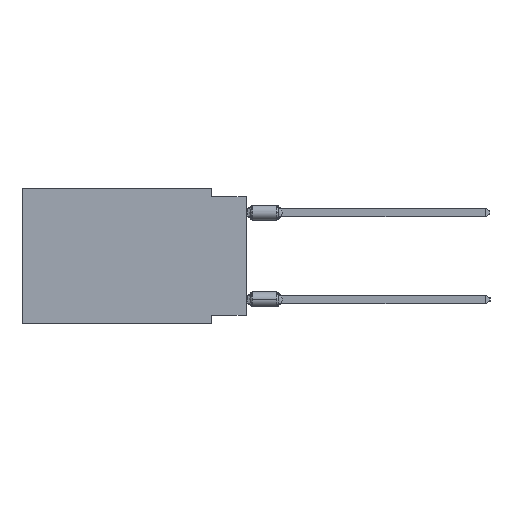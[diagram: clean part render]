
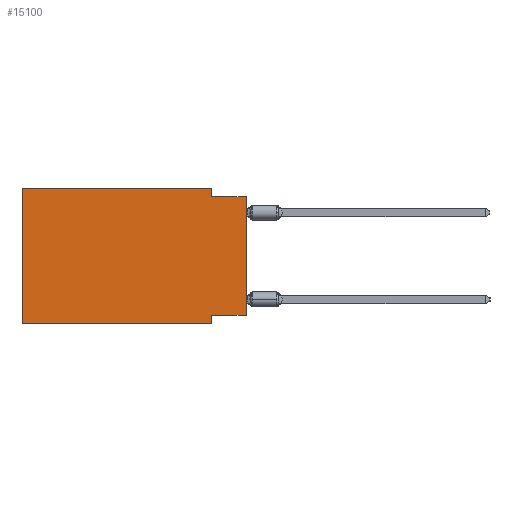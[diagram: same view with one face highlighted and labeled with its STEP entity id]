
A CAD part, left-side view. The second image highlights one B-rep face of the part: STEP entity #15100.
In plain terms, the highlighted planar face has unit normal (-1, 0, 0).
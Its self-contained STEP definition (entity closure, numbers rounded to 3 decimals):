
#609 = LINE ( 'NONE', #11092, #6126 ) ;
#637 = LINE ( 'NONE', #15640, #22141 ) ;
#1046 = VERTEX_POINT ( 'NONE', #30726 ) ;
#1309 = DIRECTION ( 'NONE',  ( 0., 0., 1. ) ) ;
#1723 = LINE ( 'NONE', #22529, #19626 ) ;
#3547 = VERTEX_POINT ( 'NONE', #27599 ) ;
#3715 = EDGE_CURVE ( 'NONE', #22138, #19962, #637, .T. ) ;
#4465 = DIRECTION ( 'NONE',  ( 0., -1., 0. ) ) ;
#4510 = VECTOR ( 'NONE', #1309, 1000. ) ;
#5975 = ORIENTED_EDGE ( 'NONE', *, *, #26621, .F. ) ;
#6126 = VECTOR ( 'NONE', #20151, 1000. ) ;
#6165 = DIRECTION ( 'NONE',  ( 0., 1., 0. ) ) ;
#6294 = EDGE_CURVE ( 'NONE', #22138, #8453, #24699, .T. ) ;
#7339 = ORIENTED_EDGE ( 'NONE', *, *, #3715, .T. ) ;
#7971 = EDGE_CURVE ( 'NONE', #3547, #11430, #24316, .T. ) ;
#8399 = LINE ( 'NONE', #32108, #19657 ) ;
#8453 = VERTEX_POINT ( 'NONE', #26685 ) ;
#9452 = ORIENTED_EDGE ( 'NONE', *, *, #14003, .F. ) ;
#10922 = ORIENTED_EDGE ( 'NONE', *, *, #25157, .F. ) ;
#11092 = CARTESIAN_POINT ( 'NONE',  ( 0., 0., 0. ) ) ;
#11134 = CARTESIAN_POINT ( 'NONE',  ( 0., 16.383, 0. ) ) ;
#11430 = VERTEX_POINT ( 'NONE', #21937 ) ;
#11693 = CARTESIAN_POINT ( 'NONE',  ( 0., 16.383, -9.906 ) ) ;
#13054 = VECTOR ( 'NONE', #6165, 1000. ) ;
#14003 = EDGE_CURVE ( 'NONE', #1046, #33826, #18894, .T. ) ;
#14511 = VERTEX_POINT ( 'NONE', #32408 ) ;
#15100 = ADVANCED_FACE ( 'NONE', ( #18068 ), #28532, .F. ) ;
#15464 = DIRECTION ( 'NONE',  ( 1., 0., 0. ) ) ;
#15640 = CARTESIAN_POINT ( 'NONE',  ( 0., 16.383, -9.906 ) ) ;
#15769 = AXIS2_PLACEMENT_3D ( 'NONE', #28194, #15464, #33014 ) ;
#17834 = CARTESIAN_POINT ( 'NONE',  ( 0., 2.54, -9.271 ) ) ;
#17922 = VECTOR ( 'NONE', #29975, 1000. ) ;
#18068 = FACE_OUTER_BOUND ( 'NONE', #26609, .T. ) ;
#18894 = LINE ( 'NONE', #32446, #13054 ) ;
#19154 = CARTESIAN_POINT ( 'NONE',  ( 0., 0., -0.635 ) ) ;
#19626 = VECTOR ( 'NONE', #4465, 1000. ) ;
#19657 = VECTOR ( 'NONE', #26785, 1000. ) ;
#19962 = VERTEX_POINT ( 'NONE', #30139 ) ;
#19992 = ORIENTED_EDGE ( 'NONE', *, *, #6294, .F. ) ;
#20151 = DIRECTION ( 'NONE',  ( 0., 0., 1. ) ) ;
#21729 = DIRECTION ( 'NONE',  ( 0., -1., 0. ) ) ;
#21925 = ORIENTED_EDGE ( 'NONE', *, *, #32886, .T. ) ;
#21937 = CARTESIAN_POINT ( 'NONE',  ( 0., 0., -0.635 ) ) ;
#22106 = LINE ( 'NONE', #24845, #17922 ) ;
#22138 = VERTEX_POINT ( 'NONE', #11693 ) ;
#22141 = VECTOR ( 'NONE', #27104, 1000. ) ;
#22489 = EDGE_CURVE ( 'NONE', #14511, #3547, #22106, .T. ) ;
#22529 = CARTESIAN_POINT ( 'NONE',  ( 0., 16.383, 0. ) ) ;
#24316 = LINE ( 'NONE', #19154, #27538 ) ;
#24699 = LINE ( 'NONE', #11134, #4510 ) ;
#24845 = CARTESIAN_POINT ( 'NONE',  ( 0., 2.54, 0. ) ) ;
#25157 = EDGE_CURVE ( 'NONE', #33826, #19962, #8399, .T. ) ;
#25513 = ORIENTED_EDGE ( 'NONE', *, *, #22489, .F. ) ;
#26609 = EDGE_LOOP ( 'NONE', ( #21925, #30698, #25513, #5975, #19992, #7339, #10922, #9452 ) ) ;
#26621 = EDGE_CURVE ( 'NONE', #8453, #14511, #1723, .T. ) ;
#26685 = CARTESIAN_POINT ( 'NONE',  ( 0., 16.383, 0. ) ) ;
#26785 = DIRECTION ( 'NONE',  ( 0., 0., -1. ) ) ;
#27104 = DIRECTION ( 'NONE',  ( 0., -1., 0. ) ) ;
#27538 = VECTOR ( 'NONE', #21729, 1000. ) ;
#27599 = CARTESIAN_POINT ( 'NONE',  ( 0., 2.54, -0.635 ) ) ;
#28194 = CARTESIAN_POINT ( 'NONE',  ( 0., 16.383, 0. ) ) ;
#28532 = PLANE ( 'NONE',  #15769 ) ;
#29975 = DIRECTION ( 'NONE',  ( 0., 0., -1. ) ) ;
#30139 = CARTESIAN_POINT ( 'NONE',  ( 0., 2.54, -9.906 ) ) ;
#30698 = ORIENTED_EDGE ( 'NONE', *, *, #7971, .F. ) ;
#30726 = CARTESIAN_POINT ( 'NONE',  ( 0., 0., -9.271 ) ) ;
#32108 = CARTESIAN_POINT ( 'NONE',  ( 0., 2.54, -9.906 ) ) ;
#32408 = CARTESIAN_POINT ( 'NONE',  ( 0., 2.54, 0. ) ) ;
#32446 = CARTESIAN_POINT ( 'NONE',  ( 0., 0., -9.271 ) ) ;
#32886 = EDGE_CURVE ( 'NONE', #1046, #11430, #609, .T. ) ;
#33014 = DIRECTION ( 'NONE',  ( 0., 0., -1. ) ) ;
#33826 = VERTEX_POINT ( 'NONE', #17834 ) ;
